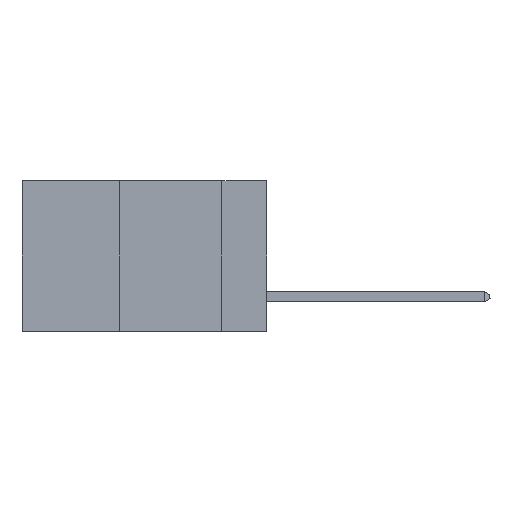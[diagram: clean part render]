
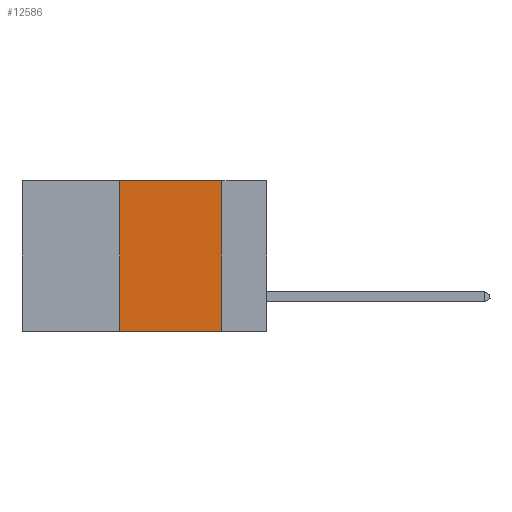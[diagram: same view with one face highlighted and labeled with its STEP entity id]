
A CAD part, left-side view. The second image highlights one B-rep face of the part: STEP entity #12586.
In plain terms, the highlighted planar face has unit normal (-1, 0, 0).
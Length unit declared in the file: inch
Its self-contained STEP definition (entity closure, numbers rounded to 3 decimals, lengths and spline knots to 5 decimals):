
#172 = CARTESIAN_POINT ( 'NONE',  ( 0., 0.11, 0. ) ) ;
#371 = DIRECTION ( 'NONE',  ( 0., -1., 0. ) ) ;
#617 = CARTESIAN_POINT ( 'NONE',  ( 0., 0.6, 0. ) ) ;
#1025 = EDGE_CURVE ( 'NONE', #9176, #11334, #7985, .T. ) ;
#1246 = EDGE_LOOP ( 'NONE', ( #5750, #8773, #13692, #4360 ) ) ;
#1596 = VERTEX_POINT ( 'NONE', #4980 ) ;
#1762 = EDGE_CURVE ( 'NONE', #1596, #9176, #14278, .T. ) ;
#2607 = CARTESIAN_POINT ( 'NONE',  ( 0., 0.6, -0.37 ) ) ;
#2608 = LINE ( 'NONE', #2607, #12851 ) ;
#3946 = PLANE ( 'NONE',  #10242 ) ;
#4234 = CARTESIAN_POINT ( 'NONE',  ( 0., 0.36, -0.37 ) ) ;
#4360 = ORIENTED_EDGE ( 'NONE', *, *, #12433, .T. ) ;
#4980 = CARTESIAN_POINT ( 'NONE',  ( 0., 0.36, 0. ) ) ;
#5404 = VERTEX_POINT ( 'NONE', #4234 ) ;
#5518 = EDGE_CURVE ( 'NONE', #5404, #1596, #12580, .T. ) ;
#5750 = ORIENTED_EDGE ( 'NONE', *, *, #1025, .F. ) ;
#6180 = DIRECTION ( 'NONE',  ( 0., 0., -1. ) ) ;
#6217 = CARTESIAN_POINT ( 'NONE',  ( 0., 0.11, -0.37 ) ) ;
#6609 = DIRECTION ( 'NONE',  ( 0., 0., 1. ) ) ;
#7233 = VECTOR ( 'NONE', #7664, 39.37008 ) ;
#7351 = CARTESIAN_POINT ( 'NONE',  ( 0., 0.36, 0. ) ) ;
#7664 = DIRECTION ( 'NONE',  ( 0., -1., 0. ) ) ;
#7814 = VECTOR ( 'NONE', #9111, 39.37008 ) ;
#7985 = LINE ( 'NONE', #172, #7814 ) ;
#8773 = ORIENTED_EDGE ( 'NONE', *, *, #1762, .F. ) ;
#9111 = DIRECTION ( 'NONE',  ( 0., 0., -1. ) ) ;
#9176 = VERTEX_POINT ( 'NONE', #14320 ) ;
#9741 = VECTOR ( 'NONE', #6609, 39.37008 ) ;
#10242 = AXIS2_PLACEMENT_3D ( 'NONE', #617, #13971, #6180 ) ;
#11334 = VERTEX_POINT ( 'NONE', #6217 ) ;
#11599 = FACE_OUTER_BOUND ( 'NONE', #1246, .T. ) ;
#12433 = EDGE_CURVE ( 'NONE', #5404, #11334, #2608, .T. ) ;
#12580 = LINE ( 'NONE', #7351, #9741 ) ;
#12586 = ADVANCED_FACE ( 'NONE', ( #11599 ), #3946, .F. ) ;
#12851 = VECTOR ( 'NONE', #371, 39.37008 ) ;
#13692 = ORIENTED_EDGE ( 'NONE', *, *, #5518, .F. ) ;
#13971 = DIRECTION ( 'NONE',  ( 1., 0., 0. ) ) ;
#14278 = LINE ( 'NONE', #14391, #7233 ) ;
#14320 = CARTESIAN_POINT ( 'NONE',  ( 0., 0.11, 0. ) ) ;
#14391 = CARTESIAN_POINT ( 'NONE',  ( 0., 0.6, 0. ) ) ;
